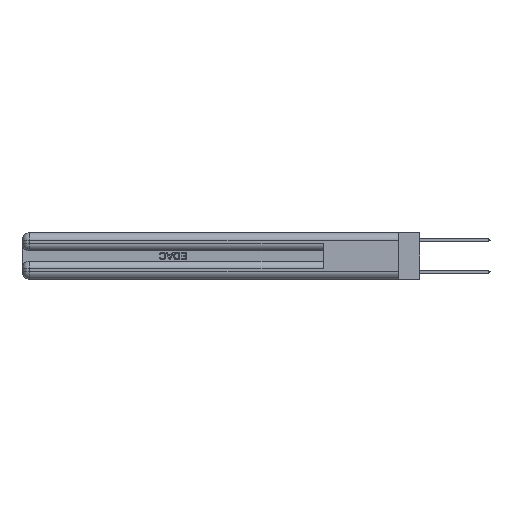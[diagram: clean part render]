
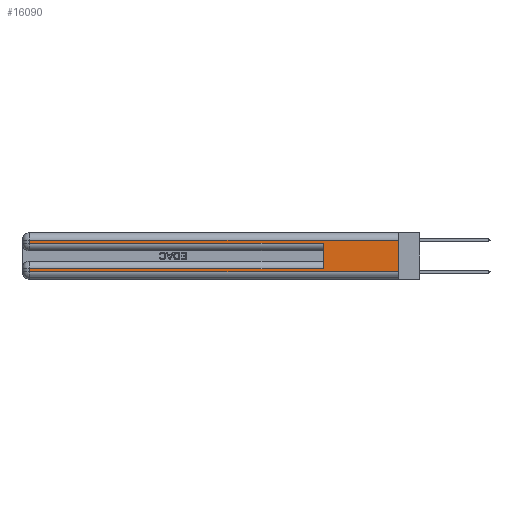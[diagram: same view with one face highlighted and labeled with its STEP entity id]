
A CAD part, left-side view. The second image highlights one B-rep face of the part: STEP entity #16090.
In plain terms, the highlighted planar face has unit normal (-1, 0, 0).
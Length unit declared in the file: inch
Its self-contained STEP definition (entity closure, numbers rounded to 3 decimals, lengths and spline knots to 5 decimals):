
#487 = EDGE_CURVE ( 'NONE', #31981, #23072, #14402, .T. ) ;
#752 = VERTEX_POINT ( 'NONE', #31942 ) ;
#979 = LINE ( 'NONE', #12579, #32176 ) ;
#1197 = EDGE_CURVE ( 'NONE', #18606, #13630, #34303, .T. ) ;
#1260 = EDGE_CURVE ( 'NONE', #752, #36012, #6156, .T. ) ;
#2865 = CARTESIAN_POINT ( 'NONE',  ( 0., 0., 0.06 ) ) ;
#3861 = CARTESIAN_POINT ( 'NONE',  ( 0., 0.6, 0.285 ) ) ;
#6156 = LINE ( 'NONE', #20350, #12942 ) ;
#6274 = DIRECTION ( 'NONE',  ( 1., 0., 0. ) ) ;
#6405 = DIRECTION ( 'NONE',  ( 0., 0., -1. ) ) ;
#6626 = LINE ( 'NONE', #20612, #20116 ) ;
#6630 = EDGE_CURVE ( 'NONE', #34336, #23072, #31604, .T. ) ;
#7174 = ORIENTED_EDGE ( 'NONE', *, *, #15345, .F. ) ;
#8063 = ORIENTED_EDGE ( 'NONE', *, *, #25429, .T. ) ;
#8421 = CARTESIAN_POINT ( 'NONE',  ( 0., 0.6, 0.085 ) ) ;
#8726 = VECTOR ( 'NONE', #20157, 39.37008 ) ;
#8820 = EDGE_CURVE ( 'NONE', #36012, #31981, #6626, .T. ) ;
#9064 = FACE_OUTER_BOUND ( 'NONE', #17987, .T. ) ;
#9763 = CARTESIAN_POINT ( 'NONE',  ( 0., 2.94, 0.31 ) ) ;
#10108 = LINE ( 'NONE', #24131, #30417 ) ;
#11557 = CARTESIAN_POINT ( 'NONE',  ( 0., 2.94, 0.37 ) ) ;
#12579 = CARTESIAN_POINT ( 'NONE',  ( 0., 0., 0.37 ) ) ;
#12942 = VECTOR ( 'NONE', #29994, 39.37008 ) ;
#13630 = VERTEX_POINT ( 'NONE', #26933 ) ;
#14254 = LINE ( 'NONE', #2865, #35784 ) ;
#14402 = LINE ( 'NONE', #34178, #15276 ) ;
#15019 = DIRECTION ( 'NONE',  ( 0., 0., -1. ) ) ;
#15276 = VECTOR ( 'NONE', #25809, 39.37008 ) ;
#15325 = DIRECTION ( 'NONE',  ( 0., -1., 0. ) ) ;
#15345 = EDGE_CURVE ( 'NONE', #752, #27633, #979, .T. ) ;
#16090 = ADVANCED_FACE ( 'NONE', ( #9064 ), #17851, .F. ) ;
#17851 = PLANE ( 'NONE',  #27475 ) ;
#17987 = EDGE_LOOP ( 'NONE', ( #7174, #25595, #22805, #18468, #32979, #8063, #30066, #28924 ) ) ;
#18327 = CARTESIAN_POINT ( 'NONE',  ( 0., 2.94, 0.285 ) ) ;
#18468 = ORIENTED_EDGE ( 'NONE', *, *, #487, .T. ) ;
#18606 = VERTEX_POINT ( 'NONE', #19507 ) ;
#19507 = CARTESIAN_POINT ( 'NONE',  ( 0., 2.94, 0.085 ) ) ;
#20009 = VECTOR ( 'NONE', #31784, 39.37008 ) ;
#20116 = VECTOR ( 'NONE', #15019, 39.37008 ) ;
#20157 = DIRECTION ( 'NONE',  ( 0., 0., -1. ) ) ;
#20281 = CARTESIAN_POINT ( 'NONE',  ( 0., 0., 0.37 ) ) ;
#20350 = CARTESIAN_POINT ( 'NONE',  ( 0., 0., 0.31 ) ) ;
#20612 = CARTESIAN_POINT ( 'NONE',  ( 0., 2.94, 0.37 ) ) ;
#22805 = ORIENTED_EDGE ( 'NONE', *, *, #8820, .T. ) ;
#23072 = VERTEX_POINT ( 'NONE', #3861 ) ;
#24131 = CARTESIAN_POINT ( 'NONE',  ( 0., 0., 0.085 ) ) ;
#25429 = EDGE_CURVE ( 'NONE', #34336, #18606, #10108, .T. ) ;
#25595 = ORIENTED_EDGE ( 'NONE', *, *, #1260, .T. ) ;
#25809 = DIRECTION ( 'NONE',  ( 0., -1., 0. ) ) ;
#25876 = DIRECTION ( 'NONE',  ( 0., 0., -1. ) ) ;
#26933 = CARTESIAN_POINT ( 'NONE',  ( 0., 2.94, 0.06 ) ) ;
#27475 = AXIS2_PLACEMENT_3D ( 'NONE', #20281, #6274, #25876 ) ;
#27633 = VERTEX_POINT ( 'NONE', #28313 ) ;
#28194 = EDGE_CURVE ( 'NONE', #13630, #27633, #14254, .T. ) ;
#28313 = CARTESIAN_POINT ( 'NONE',  ( 0., 0., 0.06 ) ) ;
#28924 = ORIENTED_EDGE ( 'NONE', *, *, #28194, .T. ) ;
#29741 = DIRECTION ( 'NONE',  ( 0., 1., 0. ) ) ;
#29994 = DIRECTION ( 'NONE',  ( 0., 1., 0. ) ) ;
#30066 = ORIENTED_EDGE ( 'NONE', *, *, #1197, .T. ) ;
#30417 = VECTOR ( 'NONE', #29741, 39.37008 ) ;
#31246 = CARTESIAN_POINT ( 'NONE',  ( 0., 0.6, 0.145 ) ) ;
#31604 = LINE ( 'NONE', #31246, #20009 ) ;
#31784 = DIRECTION ( 'NONE',  ( 0., 0., 1. ) ) ;
#31942 = CARTESIAN_POINT ( 'NONE',  ( 0., 0., 0.31 ) ) ;
#31981 = VERTEX_POINT ( 'NONE', #18327 ) ;
#32176 = VECTOR ( 'NONE', #6405, 39.37008 ) ;
#32979 = ORIENTED_EDGE ( 'NONE', *, *, #6630, .F. ) ;
#34178 = CARTESIAN_POINT ( 'NONE',  ( 0., 0., 0.285 ) ) ;
#34303 = LINE ( 'NONE', #11557, #8726 ) ;
#34336 = VERTEX_POINT ( 'NONE', #8421 ) ;
#35784 = VECTOR ( 'NONE', #15325, 39.37008 ) ;
#36012 = VERTEX_POINT ( 'NONE', #9763 ) ;
